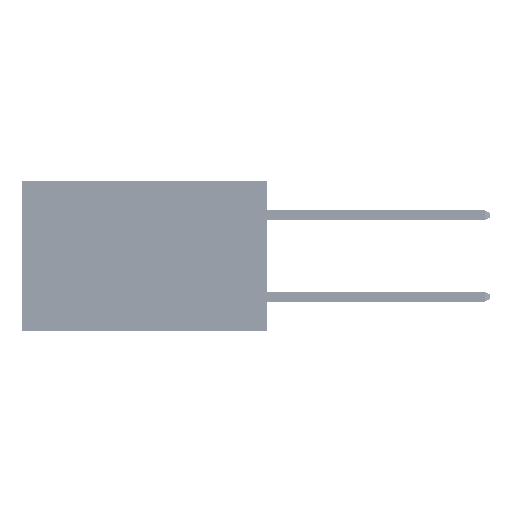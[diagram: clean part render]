
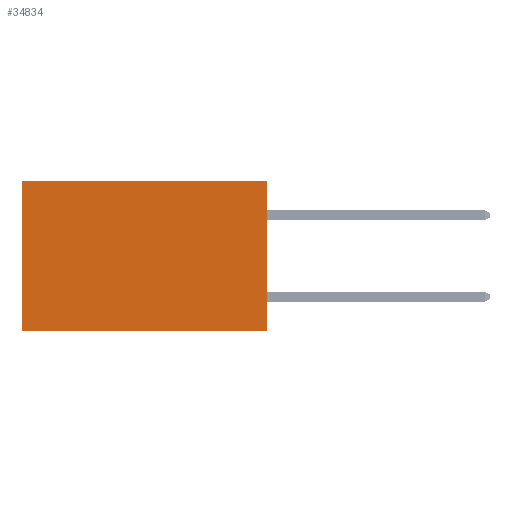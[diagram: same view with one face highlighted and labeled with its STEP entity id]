
A CAD part, left-side view. The second image highlights one B-rep face of the part: STEP entity #34834.
In plain terms, the highlighted planar face has unit normal (-1, 0, 0).
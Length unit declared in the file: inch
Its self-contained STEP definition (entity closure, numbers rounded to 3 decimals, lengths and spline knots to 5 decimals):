
#3153 = DIRECTION ( 'NONE',  ( 0., 0., -1. ) ) ;
#4897 = DIRECTION ( 'NONE',  ( 0., 1., 0. ) ) ;
#6001 = DIRECTION ( 'NONE',  ( 1., 0., 0. ) ) ;
#7157 = VERTEX_POINT ( 'NONE', #32502 ) ;
#7195 = ORIENTED_EDGE ( 'NONE', *, *, #28504, .T. ) ;
#7467 = VECTOR ( 'NONE', #10070, 39.37008 ) ;
#10070 = DIRECTION ( 'NONE',  ( 0., 1., 0. ) ) ;
#10735 = VECTOR ( 'NONE', #3153, 39.37008 ) ;
#11215 = ORIENTED_EDGE ( 'NONE', *, *, #19804, .F. ) ;
#17678 = VECTOR ( 'NONE', #33515, 39.37008 ) ;
#18472 = CARTESIAN_POINT ( 'NONE',  ( 0.2875, 0.6, 0. ) ) ;
#19804 = EDGE_CURVE ( 'NONE', #46853, #22839, #43580, .T. ) ;
#20048 = CARTESIAN_POINT ( 'NONE',  ( 0.2875, 0., 0. ) ) ;
#20390 = VERTEX_POINT ( 'NONE', #43400 ) ;
#22828 = EDGE_CURVE ( 'NONE', #7157, #22839, #28829, .T. ) ;
#22839 = VERTEX_POINT ( 'NONE', #40687 ) ;
#26232 = LINE ( 'NONE', #20048, #28054 ) ;
#28054 = VECTOR ( 'NONE', #4897, 39.37008 ) ;
#28156 = CARTESIAN_POINT ( 'NONE',  ( 0.2875, 0., -0.37 ) ) ;
#28504 = EDGE_CURVE ( 'NONE', #20390, #7157, #26232, .T. ) ;
#28820 = CARTESIAN_POINT ( 'NONE',  ( 0.2875, 0., 0. ) ) ;
#28829 = LINE ( 'NONE', #18472, #10735 ) ;
#32460 = EDGE_LOOP ( 'NONE', ( #47936, #11215, #45641, #7195 ) ) ;
#32502 = CARTESIAN_POINT ( 'NONE',  ( 0.2875, 0.6, 0. ) ) ;
#33192 = CARTESIAN_POINT ( 'NONE',  ( 0.2875, 0., 0. ) ) ;
#33515 = DIRECTION ( 'NONE',  ( 0., 0., -1. ) ) ;
#34276 = CARTESIAN_POINT ( 'NONE',  ( 0.2875, 0., -0.37 ) ) ;
#34834 = ADVANCED_FACE ( 'NONE', ( #34952 ), #35980, .F. ) ;
#34952 = FACE_OUTER_BOUND ( 'NONE', #32460, .T. ) ;
#35980 = PLANE ( 'NONE',  #45095 ) ;
#37514 = LINE ( 'NONE', #33192, #17678 ) ;
#40687 = CARTESIAN_POINT ( 'NONE',  ( 0.2875, 0.6, -0.37 ) ) ;
#43400 = CARTESIAN_POINT ( 'NONE',  ( 0.2875, 0., 0. ) ) ;
#43461 = DIRECTION ( 'NONE',  ( 0., 0., -1. ) ) ;
#43580 = LINE ( 'NONE', #28156, #7467 ) ;
#45095 = AXIS2_PLACEMENT_3D ( 'NONE', #28820, #6001, #43461 ) ;
#45641 = ORIENTED_EDGE ( 'NONE', *, *, #47413, .F. ) ;
#46853 = VERTEX_POINT ( 'NONE', #34276 ) ;
#47413 = EDGE_CURVE ( 'NONE', #20390, #46853, #37514, .T. ) ;
#47936 = ORIENTED_EDGE ( 'NONE', *, *, #22828, .T. ) ;
